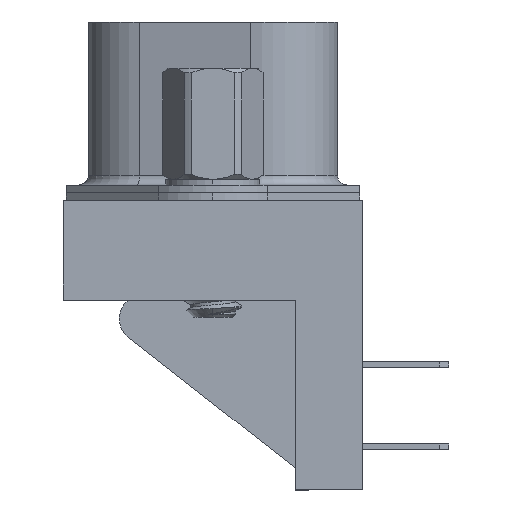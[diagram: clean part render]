
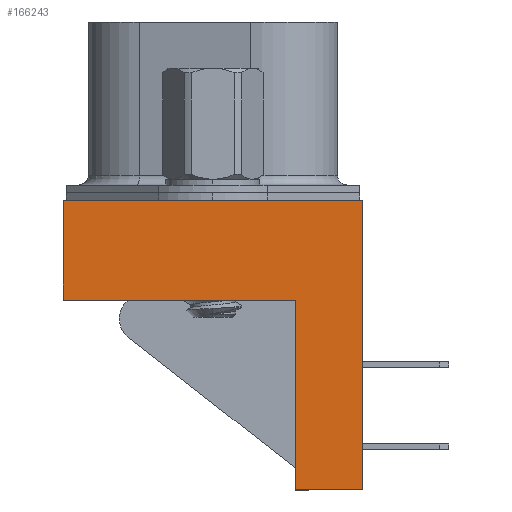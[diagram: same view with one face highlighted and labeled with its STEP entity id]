
A CAD part, left-side view. The second image highlights one B-rep face of the part: STEP entity #166243.
In plain terms, the highlighted planar face has unit normal (-1, 0, 0).
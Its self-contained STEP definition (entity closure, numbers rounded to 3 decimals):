
#3026 = LINE ( 'NONE', #33714, #59941 ) ;
#5858 = CARTESIAN_POINT ( 'NONE',  ( -4.125, 7.8, -15.1 ) ) ;
#9687 = VECTOR ( 'NONE', #124143, 1000. ) ;
#14610 = AXIS2_PLACEMENT_3D ( 'NONE', #5858, #20708, #147051 ) ;
#15991 = EDGE_CURVE ( 'NONE', #40402, #137891, #24973, .T. ) ;
#17271 = CARTESIAN_POINT ( 'NONE',  ( -4.125, 7.8, -5.2 ) ) ;
#18983 = EDGE_CURVE ( 'NONE', #160308, #163027, #142622, .T. ) ;
#19799 = PLANE ( 'NONE',  #14610 ) ;
#20708 = DIRECTION ( 'NONE',  ( -1., 0., 0. ) ) ;
#22798 = EDGE_CURVE ( 'NONE', #65233, #100887, #156471, .T. ) ;
#23791 = CARTESIAN_POINT ( 'NONE',  ( -4.125, 7.8, -15.1 ) ) ;
#24973 = LINE ( 'NONE', #129836, #56259 ) ;
#33376 = CARTESIAN_POINT ( 'NONE',  ( -4.125, -7.8, 0. ) ) ;
#33714 = CARTESIAN_POINT ( 'NONE',  ( -4.125, -7.8, -15.1 ) ) ;
#40402 = VERTEX_POINT ( 'NONE', #129062 ) ;
#46655 = VECTOR ( 'NONE', #52471, 1000. ) ;
#51747 = CARTESIAN_POINT ( 'NONE',  ( -4.125, -7.8, -15.1 ) ) ;
#52471 = DIRECTION ( 'NONE',  ( 0., 0., 1. ) ) ;
#56259 = VECTOR ( 'NONE', #85313, 1000. ) ;
#59941 = VECTOR ( 'NONE', #160959, 1000. ) ;
#65233 = VERTEX_POINT ( 'NONE', #123293 ) ;
#71169 = VECTOR ( 'NONE', #83218, 1000. ) ;
#74534 = ORIENTED_EDGE ( 'NONE', *, *, #18983, .F. ) ;
#83218 = DIRECTION ( 'NONE',  ( 0., 0., 1. ) ) ;
#85313 = DIRECTION ( 'NONE',  ( 0., -1., 0. ) ) ;
#86741 = EDGE_CURVE ( 'NONE', #137891, #100887, #3026, .T. ) ;
#91918 = ORIENTED_EDGE ( 'NONE', *, *, #22798, .F. ) ;
#95966 = EDGE_CURVE ( 'NONE', #40402, #160308, #182506, .T. ) ;
#98768 = EDGE_CURVE ( 'NONE', #163027, #65233, #181715, .T. ) ;
#99849 = DIRECTION ( 'NONE',  ( 0., -1., 0. ) ) ;
#100887 = VERTEX_POINT ( 'NONE', #33376 ) ;
#104686 = CARTESIAN_POINT ( 'NONE',  ( -4.125, -4.3, -5.2 ) ) ;
#106224 = FACE_OUTER_BOUND ( 'NONE', #136239, .T. ) ;
#116161 = VECTOR ( 'NONE', #99849, 1000. ) ;
#121955 = ORIENTED_EDGE ( 'NONE', *, *, #98768, .F. ) ;
#123293 = CARTESIAN_POINT ( 'NONE',  ( -4.125, 7.8, 0. ) ) ;
#124143 = DIRECTION ( 'NONE',  ( 0., 1., 0. ) ) ;
#126633 = ORIENTED_EDGE ( 'NONE', *, *, #15991, .T. ) ;
#129062 = CARTESIAN_POINT ( 'NONE',  ( -4.125, -4.3, -15.1 ) ) ;
#129836 = CARTESIAN_POINT ( 'NONE',  ( -4.125, 7.8, -15.1 ) ) ;
#136239 = EDGE_LOOP ( 'NONE', ( #74534, #151357, #126633, #166955, #91918, #121955 ) ) ;
#137891 = VERTEX_POINT ( 'NONE', #51747 ) ;
#141716 = CARTESIAN_POINT ( 'NONE',  ( -4.125, 7.8, -5.2 ) ) ;
#142622 = LINE ( 'NONE', #141716, #9687 ) ;
#147051 = DIRECTION ( 'NONE',  ( 0., -1., 0. ) ) ;
#151357 = ORIENTED_EDGE ( 'NONE', *, *, #95966, .F. ) ;
#153710 = CARTESIAN_POINT ( 'NONE',  ( -4.125, 7.8, 0. ) ) ;
#156471 = LINE ( 'NONE', #153710, #116161 ) ;
#160308 = VERTEX_POINT ( 'NONE', #104686 ) ;
#160959 = DIRECTION ( 'NONE',  ( 0., 0., 1. ) ) ;
#163027 = VERTEX_POINT ( 'NONE', #17271 ) ;
#166243 = ADVANCED_FACE ( 'NONE', ( #106224 ), #19799, .T. ) ;
#166955 = ORIENTED_EDGE ( 'NONE', *, *, #86741, .T. ) ;
#167630 = CARTESIAN_POINT ( 'NONE',  ( -4.125, -4.3, -15.1 ) ) ;
#181715 = LINE ( 'NONE', #23791, #71169 ) ;
#182506 = LINE ( 'NONE', #167630, #46655 ) ;
